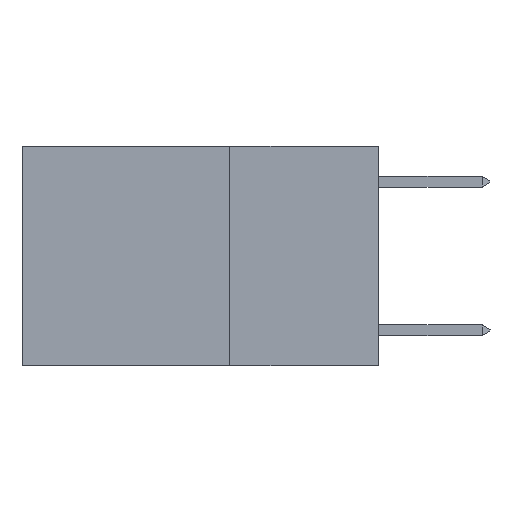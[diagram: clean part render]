
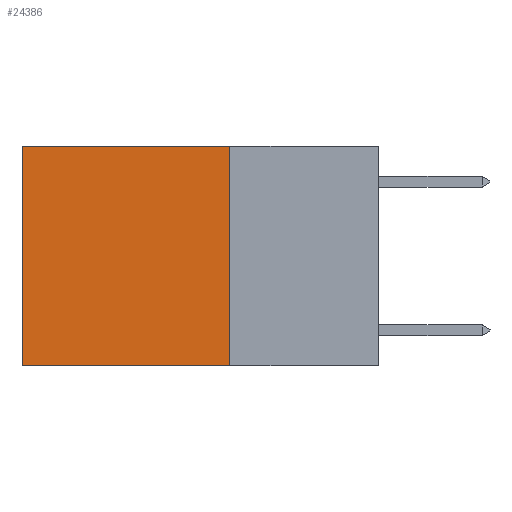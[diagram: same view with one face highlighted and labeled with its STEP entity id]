
A CAD part, left-side view. The second image highlights one B-rep face of the part: STEP entity #24386.
In plain terms, the highlighted planar face has unit normal (-1, 0, 0).
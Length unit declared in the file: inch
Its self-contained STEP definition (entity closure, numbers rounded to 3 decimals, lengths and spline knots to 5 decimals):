
#710 = FACE_OUTER_BOUND ( 'NONE', #20282, .T. ) ;
#776 = DIRECTION ( 'NONE',  ( 0., 1., 0. ) ) ;
#1065 = PLANE ( 'NONE',  #1976 ) ;
#1976 = AXIS2_PLACEMENT_3D ( 'NONE', #3499, #19403, #5792 ) ;
#2099 = VERTEX_POINT ( 'NONE', #13549 ) ;
#2187 = VECTOR ( 'NONE', #13979, 39.37008 ) ;
#2366 = LINE ( 'NONE', #9403, #2187 ) ;
#2527 = ORIENTED_EDGE ( 'NONE', *, *, #26432, .F. ) ;
#3499 = CARTESIAN_POINT ( 'NONE',  ( 0.2625, 0.25, 0. ) ) ;
#4021 = DIRECTION ( 'NONE',  ( 0., 0., -1. ) ) ;
#4596 = VERTEX_POINT ( 'NONE', #12496 ) ;
#5610 = LINE ( 'NONE', #19931, #6205 ) ;
#5792 = DIRECTION ( 'NONE',  ( 0., 0., -1. ) ) ;
#5865 = DIRECTION ( 'NONE',  ( 0., 1., 0. ) ) ;
#6205 = VECTOR ( 'NONE', #4021, 39.37008 ) ;
#6346 = LINE ( 'NONE', #16647, #28131 ) ;
#6770 = CARTESIAN_POINT ( 'NONE',  ( 0.2625, 0.25, 0. ) ) ;
#8178 = LINE ( 'NONE', #21680, #26226 ) ;
#9374 = EDGE_CURVE ( 'NONE', #10310, #4596, #5610, .T. ) ;
#9403 = CARTESIAN_POINT ( 'NONE',  ( 0.2625, 0.25, 0. ) ) ;
#9689 = EDGE_CURVE ( 'NONE', #20601, #2099, #2366, .T. ) ;
#10310 = VERTEX_POINT ( 'NONE', #22837 ) ;
#12496 = CARTESIAN_POINT ( 'NONE',  ( 0.2625, 0.6, -0.37 ) ) ;
#13549 = CARTESIAN_POINT ( 'NONE',  ( 0.2625, 0.25, -0.37 ) ) ;
#13979 = DIRECTION ( 'NONE',  ( 0., 0., -1. ) ) ;
#16647 = CARTESIAN_POINT ( 'NONE',  ( 0.2625, 0.25, -0.37 ) ) ;
#19403 = DIRECTION ( 'NONE',  ( 1., 0., 0. ) ) ;
#19931 = CARTESIAN_POINT ( 'NONE',  ( 0.2625, 0.6, 0. ) ) ;
#20282 = EDGE_LOOP ( 'NONE', ( #24744, #2527, #23824, #20469 ) ) ;
#20469 = ORIENTED_EDGE ( 'NONE', *, *, #25271, .T. ) ;
#20601 = VERTEX_POINT ( 'NONE', #6770 ) ;
#21680 = CARTESIAN_POINT ( 'NONE',  ( 0.2625, 0.25, 0. ) ) ;
#22837 = CARTESIAN_POINT ( 'NONE',  ( 0.2625, 0.6, 0. ) ) ;
#23824 = ORIENTED_EDGE ( 'NONE', *, *, #9689, .F. ) ;
#24386 = ADVANCED_FACE ( 'NONE', ( #710 ), #1065, .F. ) ;
#24744 = ORIENTED_EDGE ( 'NONE', *, *, #9374, .T. ) ;
#25271 = EDGE_CURVE ( 'NONE', #20601, #10310, #8178, .T. ) ;
#26226 = VECTOR ( 'NONE', #5865, 39.37008 ) ;
#26432 = EDGE_CURVE ( 'NONE', #2099, #4596, #6346, .T. ) ;
#28131 = VECTOR ( 'NONE', #776, 39.37008 ) ;
